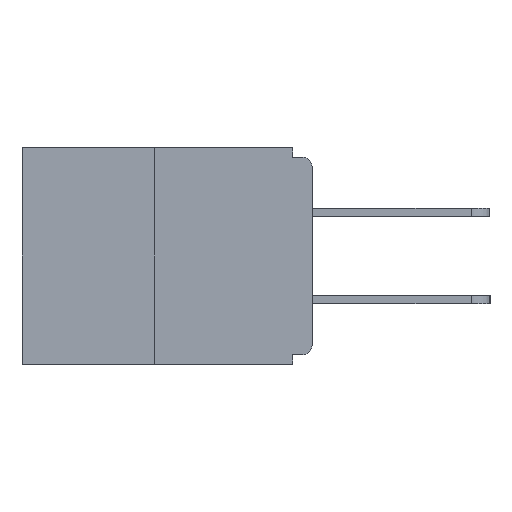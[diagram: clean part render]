
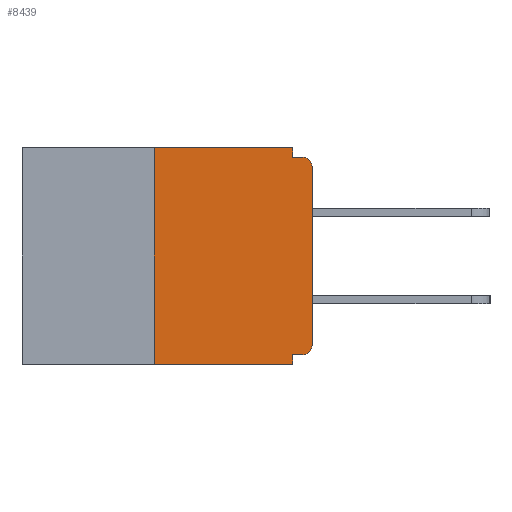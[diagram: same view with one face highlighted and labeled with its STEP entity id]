
A CAD part, left-side view. The second image highlights one B-rep face of the part: STEP entity #8439.
In plain terms, the highlighted planar face has unit normal (-1, 0, 0).
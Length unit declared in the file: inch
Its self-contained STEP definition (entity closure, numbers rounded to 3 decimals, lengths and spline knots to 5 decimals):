
#57 = EDGE_CURVE ( 'NONE', #9946, #11512, #2301, .T. ) ;
#82 = VECTOR ( 'NONE', #8824, 39.37008 ) ;
#128 = DIRECTION ( 'NONE',  ( 0., 0., -1. ) ) ;
#206 = VECTOR ( 'NONE', #9844, 39.37008 ) ;
#428 = EDGE_CURVE ( 'NONE', #3721, #795, #3453, .T. ) ;
#659 = DIRECTION ( 'NONE',  ( -1., 0., 0. ) ) ;
#693 = VERTEX_POINT ( 'NONE', #12848 ) ;
#795 = VERTEX_POINT ( 'NONE', #9158 ) ;
#924 = CARTESIAN_POINT ( 'NONE',  ( 0., 0.46, 0. ) ) ;
#1301 = EDGE_CURVE ( 'NONE', #5737, #10665, #9886, .T. ) ;
#1449 = CIRCLE ( 'NONE', #11868, 0.015 ) ;
#1578 = ORIENTED_EDGE ( 'NONE', *, *, #57, .T. ) ;
#1729 = EDGE_CURVE ( 'NONE', #693, #10531, #2699, .T. ) ;
#1816 = DIRECTION ( 'NONE',  ( 0., 0., -1. ) ) ;
#1923 = CARTESIAN_POINT ( 'NONE',  ( 0., 0., 0. ) ) ;
#2260 = CIRCLE ( 'NONE', #13203, 0.015 ) ;
#2301 = LINE ( 'NONE', #1923, #13295 ) ;
#2306 = DIRECTION ( 'NONE',  ( 1., 0., 0. ) ) ;
#2699 = LINE ( 'NONE', #9388, #6003 ) ;
#2748 = CARTESIAN_POINT ( 'NONE',  ( 0., 0.031, 0. ) ) ;
#3218 = VERTEX_POINT ( 'NONE', #11161 ) ;
#3349 = DIRECTION ( 'NONE',  ( -1., 0., 0. ) ) ;
#3453 = LINE ( 'NONE', #7045, #3799 ) ;
#3541 = CARTESIAN_POINT ( 'NONE',  ( 0., 0.031, -0.343 ) ) ;
#3721 = VERTEX_POINT ( 'NONE', #2748 ) ;
#3799 = VECTOR ( 'NONE', #6346, 39.37008 ) ;
#3967 = CARTESIAN_POINT ( 'NONE',  ( 0., 0.015, -0.313 ) ) ;
#4143 = ORIENTED_EDGE ( 'NONE', *, *, #6357, .F. ) ;
#4400 = VECTOR ( 'NONE', #11573, 39.37008 ) ;
#4906 = DIRECTION ( 'NONE',  ( 0., 0., 1. ) ) ;
#5407 = CARTESIAN_POINT ( 'NONE',  ( 0., 0.015, -0.328 ) ) ;
#5737 = VERTEX_POINT ( 'NONE', #5407 ) ;
#5749 = ORIENTED_EDGE ( 'NONE', *, *, #6950, .F. ) ;
#6003 = VECTOR ( 'NONE', #13651, 39.37008 ) ;
#6250 = CARTESIAN_POINT ( 'NONE',  ( 0., 0., -0.328 ) ) ;
#6298 = DIRECTION ( 'NONE',  ( 0., 1., 0. ) ) ;
#6346 = DIRECTION ( 'NONE',  ( 0., 0., -1. ) ) ;
#6357 = EDGE_CURVE ( 'NONE', #10665, #12075, #8743, .T. ) ;
#6489 = ORIENTED_EDGE ( 'NONE', *, *, #10302, .T. ) ;
#6669 = DIRECTION ( 'NONE',  ( 0., 0., -1. ) ) ;
#6724 = ORIENTED_EDGE ( 'NONE', *, *, #9783, .T. ) ;
#6841 = EDGE_CURVE ( 'NONE', #693, #12075, #9224, .T. ) ;
#6920 = AXIS2_PLACEMENT_3D ( 'NONE', #7735, #2306, #6669 ) ;
#6950 = EDGE_CURVE ( 'NONE', #10531, #3721, #10376, .T. ) ;
#7045 = CARTESIAN_POINT ( 'NONE',  ( 0., 0.031, 0. ) ) ;
#7561 = EDGE_LOOP ( 'NONE', ( #5749, #13224, #10589, #4143, #9182, #6489, #1578, #6724, #12414, #11396 ) ) ;
#7735 = CARTESIAN_POINT ( 'NONE',  ( 0., 0.46, 0. ) ) ;
#8338 = CARTESIAN_POINT ( 'NONE',  ( 0., 0.46, -0.343 ) ) ;
#8399 = CARTESIAN_POINT ( 'NONE',  ( 0., 0., -0.03 ) ) ;
#8439 = ADVANCED_FACE ( 'NONE', ( #10634 ), #12965, .F. ) ;
#8645 = CARTESIAN_POINT ( 'NONE',  ( 0., 0.25, 0. ) ) ;
#8719 = CARTESIAN_POINT ( 'NONE',  ( 0., 0., -0.015 ) ) ;
#8743 = LINE ( 'NONE', #12012, #82 ) ;
#8824 = DIRECTION ( 'NONE',  ( 0., 0., -1. ) ) ;
#9158 = CARTESIAN_POINT ( 'NONE',  ( 0., 0.031, -0.015 ) ) ;
#9182 = ORIENTED_EDGE ( 'NONE', *, *, #1301, .F. ) ;
#9224 = LINE ( 'NONE', #8338, #4400 ) ;
#9388 = CARTESIAN_POINT ( 'NONE',  ( 0., 0.25, 0. ) ) ;
#9536 = CARTESIAN_POINT ( 'NONE',  ( 0., 0.015, -0.03 ) ) ;
#9783 = EDGE_CURVE ( 'NONE', #11512, #3218, #1449, .T. ) ;
#9844 = DIRECTION ( 'NONE',  ( 0., -1., 0. ) ) ;
#9886 = LINE ( 'NONE', #6250, #10876 ) ;
#9946 = VERTEX_POINT ( 'NONE', #13038 ) ;
#10302 = EDGE_CURVE ( 'NONE', #5737, #9946, #2260, .T. ) ;
#10376 = LINE ( 'NONE', #924, #11050 ) ;
#10455 = DIRECTION ( 'NONE',  ( 0., -1., 0. ) ) ;
#10531 = VERTEX_POINT ( 'NONE', #8645 ) ;
#10589 = ORIENTED_EDGE ( 'NONE', *, *, #6841, .T. ) ;
#10634 = FACE_OUTER_BOUND ( 'NONE', #7561, .T. ) ;
#10665 = VERTEX_POINT ( 'NONE', #10884 ) ;
#10876 = VECTOR ( 'NONE', #6298, 39.37008 ) ;
#10884 = CARTESIAN_POINT ( 'NONE',  ( 0., 0.031, -0.328 ) ) ;
#11050 = VECTOR ( 'NONE', #10455, 39.37008 ) ;
#11161 = CARTESIAN_POINT ( 'NONE',  ( 0., 0.015, -0.015 ) ) ;
#11396 = ORIENTED_EDGE ( 'NONE', *, *, #428, .F. ) ;
#11512 = VERTEX_POINT ( 'NONE', #8399 ) ;
#11573 = DIRECTION ( 'NONE',  ( 0., -1., 0. ) ) ;
#11836 = EDGE_CURVE ( 'NONE', #795, #3218, #12051, .T. ) ;
#11868 = AXIS2_PLACEMENT_3D ( 'NONE', #9536, #3349, #128 ) ;
#12012 = CARTESIAN_POINT ( 'NONE',  ( 0., 0.031, -0.343 ) ) ;
#12051 = LINE ( 'NONE', #8719, #206 ) ;
#12075 = VERTEX_POINT ( 'NONE', #3541 ) ;
#12414 = ORIENTED_EDGE ( 'NONE', *, *, #11836, .F. ) ;
#12848 = CARTESIAN_POINT ( 'NONE',  ( 0., 0.25, -0.343 ) ) ;
#12965 = PLANE ( 'NONE',  #6920 ) ;
#13038 = CARTESIAN_POINT ( 'NONE',  ( 0., 0., -0.313 ) ) ;
#13203 = AXIS2_PLACEMENT_3D ( 'NONE', #3967, #659, #1816 ) ;
#13224 = ORIENTED_EDGE ( 'NONE', *, *, #1729, .F. ) ;
#13295 = VECTOR ( 'NONE', #4906, 39.37008 ) ;
#13651 = DIRECTION ( 'NONE',  ( 0., 0., 1. ) ) ;
